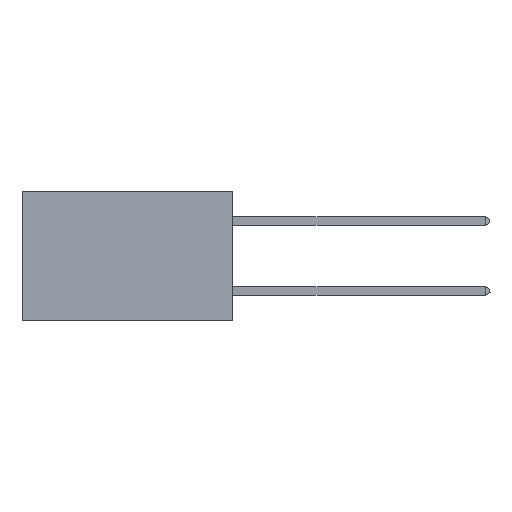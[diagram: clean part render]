
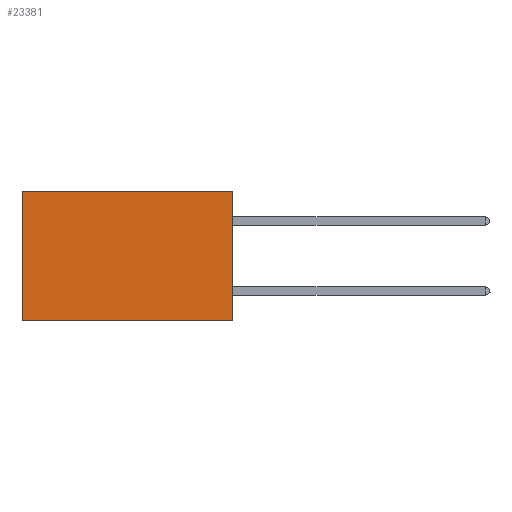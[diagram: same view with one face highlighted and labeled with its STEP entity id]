
A CAD part, left-side view. The second image highlights one B-rep face of the part: STEP entity #23381.
In plain terms, the highlighted planar face has unit normal (-1, 0, 0).
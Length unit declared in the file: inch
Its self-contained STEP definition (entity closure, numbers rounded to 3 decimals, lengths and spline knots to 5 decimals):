
#288 = ORIENTED_EDGE ( 'NONE', *, *, #8954, .T. ) ;
#392 = ORIENTED_EDGE ( 'NONE', *, *, #13917, .F. ) ;
#722 = CARTESIAN_POINT ( 'NONE',  ( 0.2875, 0., 0. ) ) ;
#1240 = VECTOR ( 'NONE', #17432, 39.37008 ) ;
#1886 = ORIENTED_EDGE ( 'NONE', *, *, #17522, .F. ) ;
#5957 = VERTEX_POINT ( 'NONE', #10848 ) ;
#6499 = DIRECTION ( 'NONE',  ( 0., 0., -1. ) ) ;
#6617 = ORIENTED_EDGE ( 'NONE', *, *, #6681, .T. ) ;
#6681 = EDGE_CURVE ( 'NONE', #5957, #20253, #25105, .T. ) ;
#8150 = EDGE_LOOP ( 'NONE', ( #288, #1886, #392, #6617 ) ) ;
#8653 = CARTESIAN_POINT ( 'NONE',  ( 0.2875, 0.6, 0. ) ) ;
#8954 = EDGE_CURVE ( 'NONE', #20253, #19310, #24043, .T. ) ;
#9159 = DIRECTION ( 'NONE',  ( 0., 0., -1. ) ) ;
#9575 = LINE ( 'NONE', #19579, #1240 ) ;
#9807 = VECTOR ( 'NONE', #9159, 39.37008 ) ;
#10406 = CARTESIAN_POINT ( 'NONE',  ( 0.2875, 0.6, -0.37 ) ) ;
#10820 = DIRECTION ( 'NONE',  ( 1., 0., 0. ) ) ;
#10848 = CARTESIAN_POINT ( 'NONE',  ( 0.2875, 0., 0. ) ) ;
#10918 = CARTESIAN_POINT ( 'NONE',  ( 0.2875, 0., 0. ) ) ;
#13850 = AXIS2_PLACEMENT_3D ( 'NONE', #10918, #10820, #20763 ) ;
#13917 = EDGE_CURVE ( 'NONE', #5957, #15676, #25359, .T. ) ;
#15676 = VERTEX_POINT ( 'NONE', #23296 ) ;
#17432 = DIRECTION ( 'NONE',  ( 0., 1., 0. ) ) ;
#17522 = EDGE_CURVE ( 'NONE', #15676, #19310, #9575, .T. ) ;
#18600 = DIRECTION ( 'NONE',  ( 0., 1., 0. ) ) ;
#18620 = FACE_OUTER_BOUND ( 'NONE', #8150, .T. ) ;
#19310 = VERTEX_POINT ( 'NONE', #10406 ) ;
#19579 = CARTESIAN_POINT ( 'NONE',  ( 0.2875, 0., -0.37 ) ) ;
#19710 = CARTESIAN_POINT ( 'NONE',  ( 0.2875, 0., 0. ) ) ;
#19807 = VECTOR ( 'NONE', #18600, 39.37008 ) ;
#20253 = VERTEX_POINT ( 'NONE', #8653 ) ;
#20754 = CARTESIAN_POINT ( 'NONE',  ( 0.2875, 0.6, 0. ) ) ;
#20763 = DIRECTION ( 'NONE',  ( 0., 0., -1. ) ) ;
#22910 = PLANE ( 'NONE',  #13850 ) ;
#23296 = CARTESIAN_POINT ( 'NONE',  ( 0.2875, 0., -0.37 ) ) ;
#23381 = ADVANCED_FACE ( 'NONE', ( #18620 ), #22910, .F. ) ;
#24043 = LINE ( 'NONE', #20754, #9807 ) ;
#24098 = VECTOR ( 'NONE', #6499, 39.37008 ) ;
#25105 = LINE ( 'NONE', #722, #19807 ) ;
#25359 = LINE ( 'NONE', #19710, #24098 ) ;
